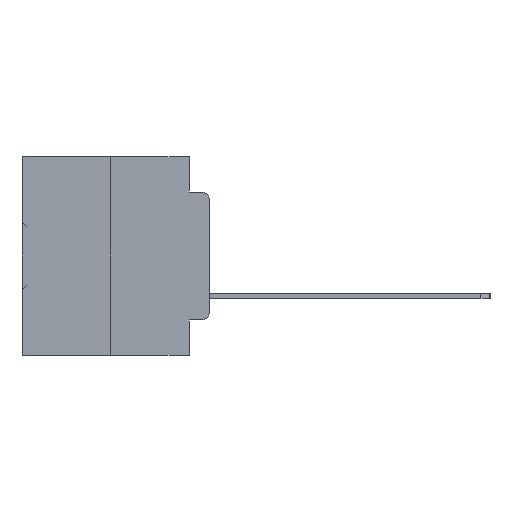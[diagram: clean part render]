
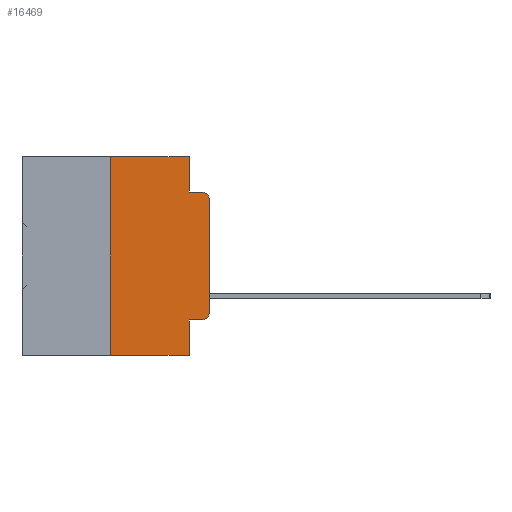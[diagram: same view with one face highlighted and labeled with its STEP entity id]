
A CAD part, left-side view. The second image highlights one B-rep face of the part: STEP entity #16469.
In plain terms, the highlighted planar face has unit normal (-1, 0, 0).
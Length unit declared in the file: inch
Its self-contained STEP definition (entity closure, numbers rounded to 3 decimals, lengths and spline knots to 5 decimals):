
#218 = ORIENTED_EDGE ( 'NONE', *, *, #30894, .T. ) ;
#700 = ORIENTED_EDGE ( 'NONE', *, *, #29555, .T. ) ;
#1552 = CARTESIAN_POINT ( 'NONE',  ( 0., 0., -0.1085 ) ) ;
#2705 = DIRECTION ( 'NONE',  ( 0., -1., 0. ) ) ;
#3333 = AXIS2_PLACEMENT_3D ( 'NONE', #10224, #30049, #13129 ) ;
#3381 = VECTOR ( 'NONE', #36332, 39.37008 ) ;
#3427 = CARTESIAN_POINT ( 'NONE',  ( 0., 0., 0. ) ) ;
#3443 = VECTOR ( 'NONE', #2705, 39.37008 ) ;
#3974 = DIRECTION ( 'NONE',  ( 0., -1., 0. ) ) ;
#5242 = CIRCLE ( 'NONE', #27535, 0.02 ) ;
#6332 = VERTEX_POINT ( 'NONE', #19859 ) ;
#6867 = EDGE_CURVE ( 'NONE', #7476, #6332, #29583, .T. ) ;
#6914 = VECTOR ( 'NONE', #24970, 39.37008 ) ;
#6996 = CARTESIAN_POINT ( 'NONE',  ( 0., 0.051, -0.4115 ) ) ;
#7382 = ORIENTED_EDGE ( 'NONE', *, *, #33439, .F. ) ;
#7476 = VERTEX_POINT ( 'NONE', #6996 ) ;
#7750 = CARTESIAN_POINT ( 'NONE',  ( 0., 0.051, 0. ) ) ;
#8643 = CARTESIAN_POINT ( 'NONE',  ( 0., 0.051, 0. ) ) ;
#8860 = CARTESIAN_POINT ( 'NONE',  ( 0., 0., -0.3915 ) ) ;
#8867 = VECTOR ( 'NONE', #32766, 39.37008 ) ;
#9646 = VECTOR ( 'NONE', #25689, 39.37008 ) ;
#10134 = CARTESIAN_POINT ( 'NONE',  ( 0., 0.25, 0. ) ) ;
#10224 = CARTESIAN_POINT ( 'NONE',  ( 0., 0.02, -0.3915 ) ) ;
#12292 = VERTEX_POINT ( 'NONE', #8860 ) ;
#12332 = ORIENTED_EDGE ( 'NONE', *, *, #35313, .F. ) ;
#13129 = DIRECTION ( 'NONE',  ( 0., 0., -1. ) ) ;
#13569 = CARTESIAN_POINT ( 'NONE',  ( 0., 0.051, -0.4115 ) ) ;
#13916 = CARTESIAN_POINT ( 'NONE',  ( 0., 0.051, 0. ) ) ;
#14117 = CARTESIAN_POINT ( 'NONE',  ( 0., 0.02, -0.1085 ) ) ;
#14218 = CARTESIAN_POINT ( 'NONE',  ( 0., 0.051, -0.5 ) ) ;
#15684 = CARTESIAN_POINT ( 'NONE',  ( 0., 0.473, 0. ) ) ;
#15782 = EDGE_CURVE ( 'NONE', #36511, #16458, #18252, .T. ) ;
#16027 = CARTESIAN_POINT ( 'NONE',  ( 0., 0.25, -0.5 ) ) ;
#16458 = VERTEX_POINT ( 'NONE', #21290 ) ;
#16469 = ADVANCED_FACE ( 'NONE', ( #29165 ), #18435, .F. ) ;
#16974 = DIRECTION ( 'NONE',  ( 0., 0., -1. ) ) ;
#17386 = LINE ( 'NONE', #10134, #8867 ) ;
#17889 = VERTEX_POINT ( 'NONE', #14218 ) ;
#18252 = LINE ( 'NONE', #26725, #25739 ) ;
#18435 = PLANE ( 'NONE',  #21281 ) ;
#18561 = DIRECTION ( 'NONE',  ( 0., 0., -1. ) ) ;
#18622 = LINE ( 'NONE', #19582, #3381 ) ;
#18685 = LINE ( 'NONE', #19835, #3443 ) ;
#19045 = ORIENTED_EDGE ( 'NONE', *, *, #15782, .F. ) ;
#19452 = VERTEX_POINT ( 'NONE', #22384 ) ;
#19582 = CARTESIAN_POINT ( 'NONE',  ( 0., 0.473, -0.5 ) ) ;
#19835 = CARTESIAN_POINT ( 'NONE',  ( 0., 0.473, 0. ) ) ;
#19859 = CARTESIAN_POINT ( 'NONE',  ( 0., 0.02, -0.4115 ) ) ;
#20823 = ORIENTED_EDGE ( 'NONE', *, *, #35695, .F. ) ;
#21281 = AXIS2_PLACEMENT_3D ( 'NONE', #15684, #35341, #18561 ) ;
#21290 = CARTESIAN_POINT ( 'NONE',  ( 0., 0.02, -0.0885 ) ) ;
#21295 = VERTEX_POINT ( 'NONE', #13916 ) ;
#22384 = CARTESIAN_POINT ( 'NONE',  ( 0., 0.25, 0. ) ) ;
#23812 = VERTEX_POINT ( 'NONE', #16027 ) ;
#24970 = DIRECTION ( 'NONE',  ( 0., -1., 0. ) ) ;
#25689 = DIRECTION ( 'NONE',  ( 0., 0., -1. ) ) ;
#25739 = VECTOR ( 'NONE', #3974, 39.37008 ) ;
#26186 = VECTOR ( 'NONE', #27642, 39.37008 ) ;
#26195 = DIRECTION ( 'NONE',  ( 0., 0., 1. ) ) ;
#26725 = CARTESIAN_POINT ( 'NONE',  ( 0., 0.051, -0.0885 ) ) ;
#27148 = EDGE_CURVE ( 'NONE', #36061, #16458, #5242, .T. ) ;
#27535 = AXIS2_PLACEMENT_3D ( 'NONE', #14117, #33786, #16974 ) ;
#27642 = DIRECTION ( 'NONE',  ( 0., 0., -1. ) ) ;
#27842 = EDGE_CURVE ( 'NONE', #7476, #17889, #32223, .T. ) ;
#28723 = ORIENTED_EDGE ( 'NONE', *, *, #32274, .T. ) ;
#29165 = FACE_OUTER_BOUND ( 'NONE', #29570, .T. ) ;
#29555 = EDGE_CURVE ( 'NONE', #23812, #17889, #18622, .T. ) ;
#29570 = EDGE_LOOP ( 'NONE', ( #218, #31318, #19045, #12332, #20823, #7382, #700, #34364, #35253, #28723 ) ) ;
#29583 = LINE ( 'NONE', #13569, #6914 ) ;
#29827 = CIRCLE ( 'NONE', #3333, 0.02 ) ;
#30049 = DIRECTION ( 'NONE',  ( -1., 0., 0. ) ) ;
#30810 = VECTOR ( 'NONE', #26195, 39.37008 ) ;
#30894 = EDGE_CURVE ( 'NONE', #12292, #36061, #32552, .T. ) ;
#31318 = ORIENTED_EDGE ( 'NONE', *, *, #27148, .T. ) ;
#31765 = CARTESIAN_POINT ( 'NONE',  ( 0., 0.051, -0.0885 ) ) ;
#31878 = LINE ( 'NONE', #7750, #26186 ) ;
#32223 = LINE ( 'NONE', #8643, #9646 ) ;
#32274 = EDGE_CURVE ( 'NONE', #6332, #12292, #29827, .T. ) ;
#32552 = LINE ( 'NONE', #3427, #30810 ) ;
#32766 = DIRECTION ( 'NONE',  ( 0., 0., 1. ) ) ;
#33439 = EDGE_CURVE ( 'NONE', #23812, #19452, #17386, .T. ) ;
#33786 = DIRECTION ( 'NONE',  ( -1., 0., 0. ) ) ;
#34364 = ORIENTED_EDGE ( 'NONE', *, *, #27842, .F. ) ;
#35253 = ORIENTED_EDGE ( 'NONE', *, *, #6867, .T. ) ;
#35313 = EDGE_CURVE ( 'NONE', #21295, #36511, #31878, .T. ) ;
#35341 = DIRECTION ( 'NONE',  ( 1., 0., 0. ) ) ;
#35695 = EDGE_CURVE ( 'NONE', #19452, #21295, #18685, .T. ) ;
#36061 = VERTEX_POINT ( 'NONE', #1552 ) ;
#36332 = DIRECTION ( 'NONE',  ( 0., -1., 0. ) ) ;
#36511 = VERTEX_POINT ( 'NONE', #31765 ) ;
